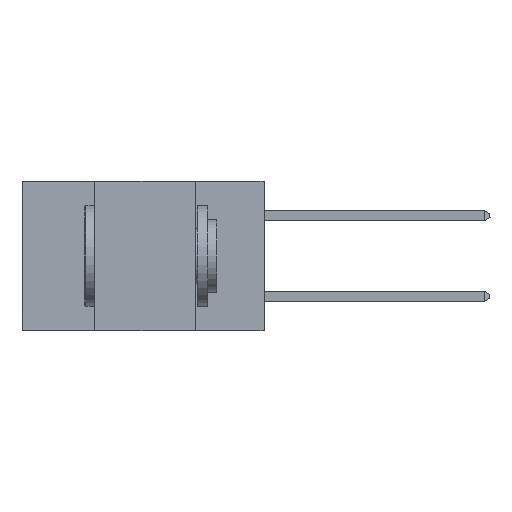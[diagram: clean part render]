
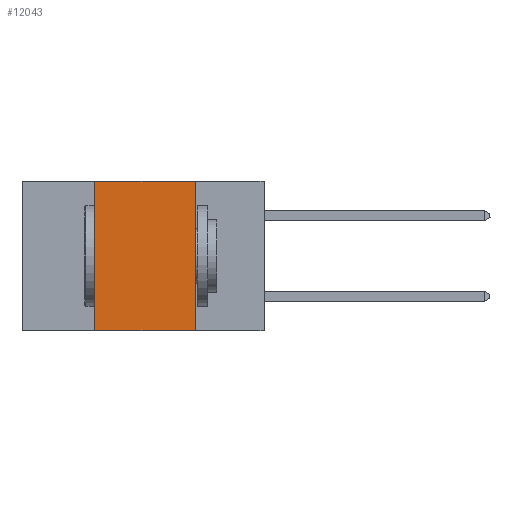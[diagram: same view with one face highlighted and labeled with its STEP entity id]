
A CAD part, left-side view. The second image highlights one B-rep face of the part: STEP entity #12043.
In plain terms, the highlighted planar face has unit normal (-1, 0, 0).
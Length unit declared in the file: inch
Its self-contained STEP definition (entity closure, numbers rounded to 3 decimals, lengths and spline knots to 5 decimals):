
#169 = ORIENTED_EDGE ( 'NONE', *, *, #12117, .F. ) ;
#286 = ORIENTED_EDGE ( 'NONE', *, *, #874, .T. ) ;
#302 = EDGE_CURVE ( 'NONE', #2218, #4051, #7058, .T. ) ;
#458 = DIRECTION ( 'NONE',  ( 1., 0., 0. ) ) ;
#874 = EDGE_CURVE ( 'NONE', #2218, #6802, #3083, .T. ) ;
#1072 = AXIS2_PLACEMENT_3D ( 'NONE', #11129, #458, #2308 ) ;
#1181 = DIRECTION ( 'NONE',  ( 0., -1., 0. ) ) ;
#1883 = VECTOR ( 'NONE', #8875, 39.37008 ) ;
#1917 = ORIENTED_EDGE ( 'NONE', *, *, #302, .F. ) ;
#2214 = EDGE_CURVE ( 'NONE', #5691, #6802, #7163, .T. ) ;
#2218 = VERTEX_POINT ( 'NONE', #3781 ) ;
#2308 = DIRECTION ( 'NONE',  ( 0., 0., -1. ) ) ;
#2334 = CARTESIAN_POINT ( 'NONE',  ( 0., 0.17, 0. ) ) ;
#2450 = FACE_OUTER_BOUND ( 'NONE', #12640, .T. ) ;
#2615 = CARTESIAN_POINT ( 'NONE',  ( 0., 0.6, 0. ) ) ;
#2927 = VECTOR ( 'NONE', #8370, 39.37008 ) ;
#3083 = LINE ( 'NONE', #6094, #10568 ) ;
#3781 = CARTESIAN_POINT ( 'NONE',  ( 0., 0.42, -0.37 ) ) ;
#4051 = VERTEX_POINT ( 'NONE', #7701 ) ;
#5017 = CARTESIAN_POINT ( 'NONE',  ( 0., 0.17, -0.37 ) ) ;
#5691 = VERTEX_POINT ( 'NONE', #8836 ) ;
#6094 = CARTESIAN_POINT ( 'NONE',  ( 0., 0.6, -0.37 ) ) ;
#6802 = VERTEX_POINT ( 'NONE', #5017 ) ;
#7058 = LINE ( 'NONE', #10695, #1883 ) ;
#7136 = PLANE ( 'NONE',  #1072 ) ;
#7163 = LINE ( 'NONE', #2334, #7783 ) ;
#7701 = CARTESIAN_POINT ( 'NONE',  ( 0., 0.42, 0. ) ) ;
#7783 = VECTOR ( 'NONE', #12263, 39.37008 ) ;
#8370 = DIRECTION ( 'NONE',  ( 0., -1., 0. ) ) ;
#8836 = CARTESIAN_POINT ( 'NONE',  ( 0., 0.17, 0. ) ) ;
#8875 = DIRECTION ( 'NONE',  ( 0., 0., 1. ) ) ;
#9297 = ORIENTED_EDGE ( 'NONE', *, *, #2214, .F. ) ;
#10568 = VECTOR ( 'NONE', #1181, 39.37008 ) ;
#10695 = CARTESIAN_POINT ( 'NONE',  ( 0., 0.42, 0. ) ) ;
#11129 = CARTESIAN_POINT ( 'NONE',  ( 0., 0.6, 0. ) ) ;
#11487 = LINE ( 'NONE', #2615, #2927 ) ;
#12043 = ADVANCED_FACE ( 'NONE', ( #2450 ), #7136, .F. ) ;
#12117 = EDGE_CURVE ( 'NONE', #4051, #5691, #11487, .T. ) ;
#12263 = DIRECTION ( 'NONE',  ( 0., 0., -1. ) ) ;
#12640 = EDGE_LOOP ( 'NONE', ( #9297, #169, #1917, #286 ) ) ;
